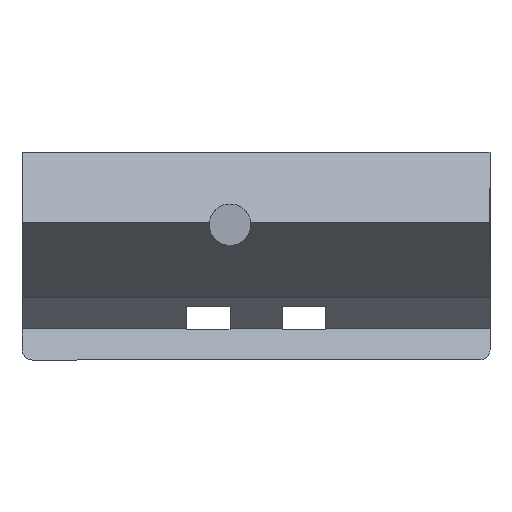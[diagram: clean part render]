
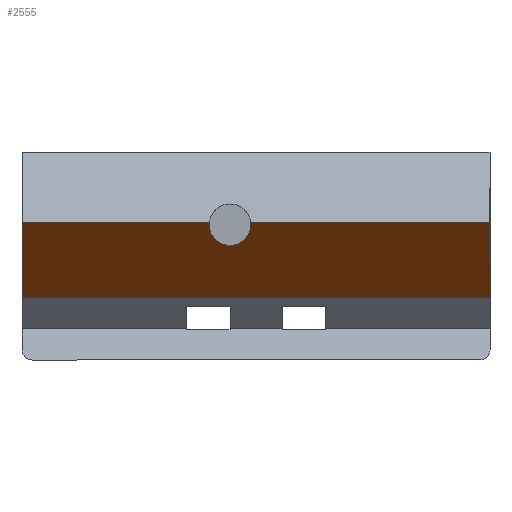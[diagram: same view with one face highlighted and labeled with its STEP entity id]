
A CAD part, left-side view. The second image highlights one B-rep face of the part: STEP entity #2555.
In plain terms, the highlighted planar face has unit normal (-0.633, 0, -0.774).
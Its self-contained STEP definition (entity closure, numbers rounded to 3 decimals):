
#44 = PLANE('',#45);
#45 = AXIS2_PLACEMENT_3D('',#46,#47,#48);
#46 = CARTESIAN_POINT('',(0.,0.,9.931));
#47 = DIRECTION('',(-0.,-1.,0.));
#48 = DIRECTION('',(0.,0.,-1.));
#158 = PLANE('',#159);
#159 = AXIS2_PLACEMENT_3D('',#160,#161,#162);
#160 = CARTESIAN_POINT('',(0.,-45.,9.931));
#161 = DIRECTION('',(-0.,-1.,0.));
#162 = DIRECTION('',(0.,0.,-1.));
#184 = PLANE('',#185);
#185 = AXIS2_PLACEMENT_3D('',#186,#187,#188);
#186 = CARTESIAN_POINT('',(-7.681,0.,23.61));
#187 = DIRECTION('',(0.774,0.,-0.633));
#188 = DIRECTION('',(-0.633,0.,-0.774));
#564 = VERTEX_POINT('',#565);
#565 = CARTESIAN_POINT('',(-16.173,0.,13.216));
#586 = EDGE_CURVE('',#564,#587,#589,.T.);
#587 = VERTEX_POINT('',#588);
#588 = CARTESIAN_POINT('',(-7.34,0.,6.));
#589 = SURFACE_CURVE('',#590,(#594,#601),.PCURVE_S1.);
#590 = LINE('',#591,#592);
#591 = CARTESIAN_POINT('',(-16.173,0.,13.216));
#592 = VECTOR('',#593,1.);
#593 = DIRECTION('',(0.774,0.,-0.633));
#594 = PCURVE('',#44,#595);
#595 = DEFINITIONAL_REPRESENTATION('',(#596),#600);
#596 = LINE('',#597,#598);
#597 = CARTESIAN_POINT('',(-3.285,-16.173));
#598 = VECTOR('',#599,1.);
#599 = DIRECTION('',(0.633,0.774));
#600 = ( GEOMETRIC_REPRESENTATION_CONTEXT(2) 
PARAMETRIC_REPRESENTATION_CONTEXT() REPRESENTATION_CONTEXT('2D SPACE',''
  ) );
#601 = PCURVE('',#602,#607);
#602 = PLANE('',#603);
#603 = AXIS2_PLACEMENT_3D('',#604,#605,#606);
#604 = CARTESIAN_POINT('',(-16.173,0.,13.216));
#605 = DIRECTION('',(0.633,0.,0.774));
#606 = DIRECTION('',(0.774,0.,-0.633));
#607 = DEFINITIONAL_REPRESENTATION('',(#608),#612);
#608 = LINE('',#609,#610);
#609 = CARTESIAN_POINT('',(0.,0.));
#610 = VECTOR('',#611,1.);
#611 = DIRECTION('',(1.,0.));
#612 = ( GEOMETRIC_REPRESENTATION_CONTEXT(2) 
PARAMETRIC_REPRESENTATION_CONTEXT() REPRESENTATION_CONTEXT('2D SPACE',''
  ) );
#630 = PLANE('',#631);
#631 = AXIS2_PLACEMENT_3D('',#632,#633,#634);
#632 = CARTESIAN_POINT('',(-9.,0.,6.));
#633 = DIRECTION('',(0.,0.,1.));
#634 = DIRECTION('',(1.,0.,0.));
#820 = VERTEX_POINT('',#821);
#821 = CARTESIAN_POINT('',(-16.173,-45.,13.216));
#842 = EDGE_CURVE('',#843,#820,#845,.T.);
#843 = VERTEX_POINT('',#844);
#844 = CARTESIAN_POINT('',(-16.173,-21.988,
    13.216));
#845 = SURFACE_CURVE('',#846,(#850,#857),.PCURVE_S1.);
#846 = LINE('',#847,#848);
#847 = CARTESIAN_POINT('',(-16.173,0.,13.216));
#848 = VECTOR('',#849,1.);
#849 = DIRECTION('',(0.,-1.,0.));
#850 = PCURVE('',#184,#851);
#851 = DEFINITIONAL_REPRESENTATION('',(#852),#856);
#852 = LINE('',#853,#854);
#853 = CARTESIAN_POINT('',(13.422,0.));
#854 = VECTOR('',#855,1.);
#855 = DIRECTION('',(0.,-1.));
#856 = ( GEOMETRIC_REPRESENTATION_CONTEXT(2) 
PARAMETRIC_REPRESENTATION_CONTEXT() REPRESENTATION_CONTEXT('2D SPACE',''
  ) );
#857 = PCURVE('',#602,#858);
#858 = DEFINITIONAL_REPRESENTATION('',(#859),#863);
#859 = LINE('',#860,#861);
#860 = CARTESIAN_POINT('',(0.,0.));
#861 = VECTOR('',#862,1.);
#862 = DIRECTION('',(0.,-1.));
#863 = ( GEOMETRIC_REPRESENTATION_CONTEXT(2) 
PARAMETRIC_REPRESENTATION_CONTEXT() REPRESENTATION_CONTEXT('2D SPACE',''
  ) );
#866 = VERTEX_POINT('',#867);
#867 = CARTESIAN_POINT('',(-16.173,-18.012,
    13.216));
#882 = CYLINDRICAL_SURFACE('',#883,2.);
#883 = AXIS2_PLACEMENT_3D('',#884,#885,#886);
#884 = CARTESIAN_POINT('',(-25.,-20.,13.));
#885 = DIRECTION('',(-1.,0.,0.));
#886 = DIRECTION('',(0.,0.,-1.));
#902 = EDGE_CURVE('',#564,#866,#903,.T.);
#903 = SURFACE_CURVE('',#904,(#908,#915),.PCURVE_S1.);
#904 = LINE('',#905,#906);
#905 = CARTESIAN_POINT('',(-16.173,0.,13.216));
#906 = VECTOR('',#907,1.);
#907 = DIRECTION('',(0.,-1.,0.));
#908 = PCURVE('',#184,#909);
#909 = DEFINITIONAL_REPRESENTATION('',(#910),#914);
#910 = LINE('',#911,#912);
#911 = CARTESIAN_POINT('',(13.422,0.));
#912 = VECTOR('',#913,1.);
#913 = DIRECTION('',(0.,-1.));
#914 = ( GEOMETRIC_REPRESENTATION_CONTEXT(2) 
PARAMETRIC_REPRESENTATION_CONTEXT() REPRESENTATION_CONTEXT('2D SPACE',''
  ) );
#915 = PCURVE('',#602,#916);
#916 = DEFINITIONAL_REPRESENTATION('',(#917),#921);
#917 = LINE('',#918,#919);
#918 = CARTESIAN_POINT('',(0.,0.));
#919 = VECTOR('',#920,1.);
#920 = DIRECTION('',(0.,-1.));
#921 = ( GEOMETRIC_REPRESENTATION_CONTEXT(2) 
PARAMETRIC_REPRESENTATION_CONTEXT() REPRESENTATION_CONTEXT('2D SPACE',''
  ) );
#1210 = EDGE_CURVE('',#1211,#820,#1213,.T.);
#1211 = VERTEX_POINT('',#1212);
#1212 = CARTESIAN_POINT('',(-7.34,-45.,6.));
#1213 = SURFACE_CURVE('',#1214,(#1218,#1225),.PCURVE_S1.);
#1214 = LINE('',#1215,#1216);
#1215 = CARTESIAN_POINT('',(-10.518,-45.,8.597));
#1216 = VECTOR('',#1217,1.);
#1217 = DIRECTION('',(-0.774,0.,0.633));
#1218 = PCURVE('',#158,#1219);
#1219 = DEFINITIONAL_REPRESENTATION('',(#1220),#1224);
#1220 = LINE('',#1221,#1222);
#1221 = CARTESIAN_POINT('',(1.335,-10.518));
#1222 = VECTOR('',#1223,1.);
#1223 = DIRECTION('',(-0.633,-0.774));
#1224 = ( GEOMETRIC_REPRESENTATION_CONTEXT(2) 
PARAMETRIC_REPRESENTATION_CONTEXT() REPRESENTATION_CONTEXT('2D SPACE',''
  ) );
#1225 = PCURVE('',#602,#1226);
#1226 = DEFINITIONAL_REPRESENTATION('',(#1227),#1231);
#1227 = LINE('',#1228,#1229);
#1228 = CARTESIAN_POINT('',(7.301,-45.));
#1229 = VECTOR('',#1230,1.);
#1230 = DIRECTION('',(-1.,0.));
#1231 = ( GEOMETRIC_REPRESENTATION_CONTEXT(2) 
PARAMETRIC_REPRESENTATION_CONTEXT() REPRESENTATION_CONTEXT('2D SPACE',''
  ) );
#2533 = EDGE_CURVE('',#1211,#587,#2534,.T.);
#2534 = SURFACE_CURVE('',#2535,(#2539,#2546),.PCURVE_S1.);
#2535 = LINE('',#2536,#2537);
#2536 = CARTESIAN_POINT('',(-7.34,0.,6.));
#2537 = VECTOR('',#2538,1.);
#2538 = DIRECTION('',(0.,1.,0.));
#2539 = PCURVE('',#630,#2540);
#2540 = DEFINITIONAL_REPRESENTATION('',(#2541),#2545);
#2541 = LINE('',#2542,#2543);
#2542 = CARTESIAN_POINT('',(1.66,0.));
#2543 = VECTOR('',#2544,1.);
#2544 = DIRECTION('',(0.,1.));
#2545 = ( GEOMETRIC_REPRESENTATION_CONTEXT(2) 
PARAMETRIC_REPRESENTATION_CONTEXT() REPRESENTATION_CONTEXT('2D SPACE',''
  ) );
#2546 = PCURVE('',#602,#2547);
#2547 = DEFINITIONAL_REPRESENTATION('',(#2548),#2552);
#2548 = LINE('',#2549,#2550);
#2549 = CARTESIAN_POINT('',(11.406,0.));
#2550 = VECTOR('',#2551,1.);
#2551 = DIRECTION('',(0.,1.));
#2552 = ( GEOMETRIC_REPRESENTATION_CONTEXT(2) 
PARAMETRIC_REPRESENTATION_CONTEXT() REPRESENTATION_CONTEXT('2D SPACE',''
  ) );
#2555 = ADVANCED_FACE('',(#2556),#602,.F.);
#2556 = FACE_BOUND('',#2557,.F.);
#2557 = EDGE_LOOP('',(#2558,#2559,#2560,#2591,#2620,#2621,#2622));
#2558 = ORIENTED_EDGE('',*,*,#586,.F.);
#2559 = ORIENTED_EDGE('',*,*,#902,.T.);
#2560 = ORIENTED_EDGE('',*,*,#2561,.F.);
#2561 = EDGE_CURVE('',#2562,#866,#2564,.T.);
#2562 = VERTEX_POINT('',#2563);
#2563 = CARTESIAN_POINT('',(-13.46,-20.,11.));
#2564 = SURFACE_CURVE('',#2565,(#2570,#2577),.PCURVE_S1.);
#2565 = ELLIPSE('',#2566,3.161,2.);
#2566 = AXIS2_PLACEMENT_3D('',#2567,#2568,#2569);
#2567 = CARTESIAN_POINT('',(-15.909,-20.,13.));
#2568 = DIRECTION('',(0.633,0.,0.774));
#2569 = DIRECTION('',(-0.774,0.,0.633
    ));
#2570 = PCURVE('',#602,#2571);
#2571 = DEFINITIONAL_REPRESENTATION('',(#2572),#2576);
#2572 = ELLIPSE('',#2573,3.161,2.);
#2573 = AXIS2_PLACEMENT_2D('',#2574,#2575);
#2574 = CARTESIAN_POINT('',(0.341,-20.));
#2575 = DIRECTION('',(-1.,0.));
#2576 = ( GEOMETRIC_REPRESENTATION_CONTEXT(2) 
PARAMETRIC_REPRESENTATION_CONTEXT() REPRESENTATION_CONTEXT('2D SPACE',''
  ) );
#2577 = PCURVE('',#882,#2578);
#2578 = DEFINITIONAL_REPRESENTATION('',(#2579),#2590);
#2579 = B_SPLINE_CURVE_WITH_KNOTS('',9,(#2580,#2581,#2582,#2583,#2584,
    #2585,#2586,#2587,#2588,#2589),.UNSPECIFIED.,.F.,.F.,(10,10),(
    3.142,5.589),.PIECEWISE_BEZIER_KNOTS.);
#2580 = CARTESIAN_POINT('',(6.283,-11.54));
#2581 = CARTESIAN_POINT('',(6.011,-11.54));
#2582 = CARTESIAN_POINT('',(5.739,-11.336));
#2583 = CARTESIAN_POINT('',(5.467,-10.929));
#2584 = CARTESIAN_POINT('',(5.196,-10.347));
#2585 = CARTESIAN_POINT('',(4.924,-9.648));
#2586 = CARTESIAN_POINT('',(4.652,-8.912));
#2587 = CARTESIAN_POINT('',(4.38,-8.218));
#2588 = CARTESIAN_POINT('',(4.108,-7.636));
#2589 = CARTESIAN_POINT('',(3.836,-7.21));
#2590 = ( GEOMETRIC_REPRESENTATION_CONTEXT(2) 
PARAMETRIC_REPRESENTATION_CONTEXT() REPRESENTATION_CONTEXT('2D SPACE',''
  ) );
#2591 = ORIENTED_EDGE('',*,*,#2592,.F.);
#2592 = EDGE_CURVE('',#843,#2562,#2593,.T.);
#2593 = SURFACE_CURVE('',#2594,(#2599,#2606),.PCURVE_S1.);
#2594 = ELLIPSE('',#2595,3.161,2.);
#2595 = AXIS2_PLACEMENT_3D('',#2596,#2597,#2598);
#2596 = CARTESIAN_POINT('',(-15.909,-20.,13.));
#2597 = DIRECTION('',(0.633,0.,0.774));
#2598 = DIRECTION('',(-0.774,0.,0.633
    ));
#2599 = PCURVE('',#602,#2600);
#2600 = DEFINITIONAL_REPRESENTATION('',(#2601),#2605);
#2601 = ELLIPSE('',#2602,3.161,2.);
#2602 = AXIS2_PLACEMENT_2D('',#2603,#2604);
#2603 = CARTESIAN_POINT('',(0.341,-20.));
#2604 = DIRECTION('',(-1.,0.));
#2605 = ( GEOMETRIC_REPRESENTATION_CONTEXT(2) 
PARAMETRIC_REPRESENTATION_CONTEXT() REPRESENTATION_CONTEXT('2D SPACE',''
  ) );
#2606 = PCURVE('',#882,#2607);
#2607 = DEFINITIONAL_REPRESENTATION('',(#2608),#2619);
#2608 = B_SPLINE_CURVE_WITH_KNOTS('',9,(#2609,#2610,#2611,#2612,#2613,
    #2614,#2615,#2616,#2617,#2618),.UNSPECIFIED.,.F.,.F.,(10,10),(
    0.694,3.142),.PIECEWISE_BEZIER_KNOTS.);
#2609 = CARTESIAN_POINT('',(2.447,-7.21));
#2610 = CARTESIAN_POINT('',(2.175,-7.636));
#2611 = CARTESIAN_POINT('',(1.903,-8.218));
#2612 = CARTESIAN_POINT('',(1.632,-8.912));
#2613 = CARTESIAN_POINT('',(1.36,-9.648));
#2614 = CARTESIAN_POINT('',(1.088,-10.347));
#2615 = CARTESIAN_POINT('',(0.816,-10.929));
#2616 = CARTESIAN_POINT('',(0.544,-11.336));
#2617 = CARTESIAN_POINT('',(0.272,-11.54));
#2618 = CARTESIAN_POINT('',(0.,-11.54));
#2619 = ( GEOMETRIC_REPRESENTATION_CONTEXT(2) 
PARAMETRIC_REPRESENTATION_CONTEXT() REPRESENTATION_CONTEXT('2D SPACE',''
  ) );
#2620 = ORIENTED_EDGE('',*,*,#842,.T.);
#2621 = ORIENTED_EDGE('',*,*,#1210,.F.);
#2622 = ORIENTED_EDGE('',*,*,#2533,.T.);
